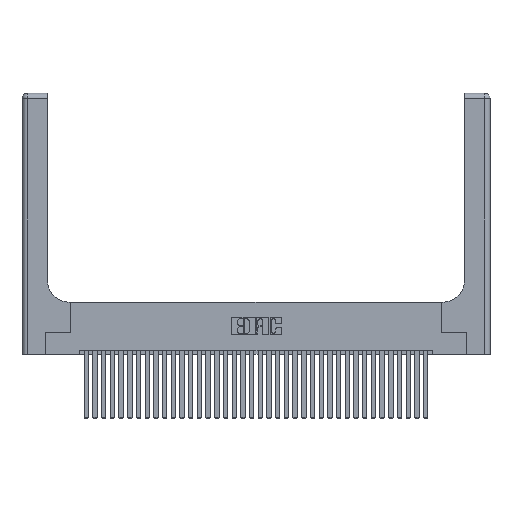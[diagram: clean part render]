
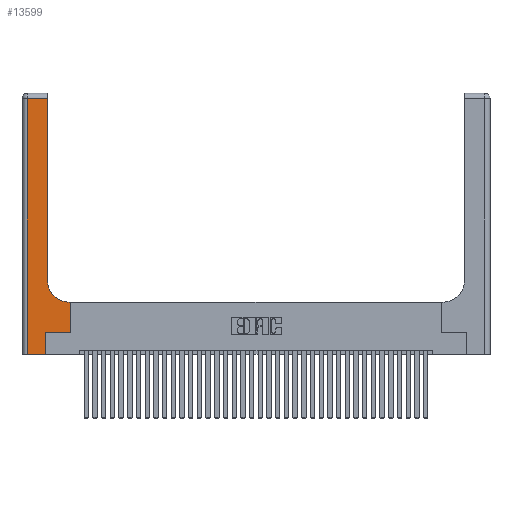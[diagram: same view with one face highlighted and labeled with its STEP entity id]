
A CAD part, top view. The second image highlights one B-rep face of the part: STEP entity #13599.
In plain terms, the highlighted planar face has unit normal (0, 0, 1).
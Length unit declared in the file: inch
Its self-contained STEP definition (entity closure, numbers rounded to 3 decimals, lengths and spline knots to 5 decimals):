
#496 = ORIENTED_EDGE ( 'NONE', *, *, #11008, .T. ) ;
#548 = CARTESIAN_POINT ( 'NONE',  ( 0.269, 0., 0.37 ) ) ;
#889 = CARTESIAN_POINT ( 'NONE',  ( 0.2915, 0.6, 0.37 ) ) ;
#1592 = LINE ( 'NONE', #29395, #14939 ) ;
#2134 = CARTESIAN_POINT ( 'NONE',  ( 0., 2.94, 0.37 ) ) ;
#2158 = EDGE_CURVE ( 'NONE', #29764, #23592, #24535, .T. ) ;
#2221 = PLANE ( 'NONE',  #5436 ) ;
#2252 = EDGE_CURVE ( 'NONE', #26574, #28063, #7174, .T. ) ;
#2369 = VECTOR ( 'NONE', #18025, 39.37008 ) ;
#3468 = CIRCLE ( 'NONE', #23201, 0.25 ) ;
#4026 = CARTESIAN_POINT ( 'NONE',  ( 0.06, 3., 0.37 ) ) ;
#4103 = DIRECTION ( 'NONE',  ( 1., 0., 0. ) ) ;
#4228 = CARTESIAN_POINT ( 'NONE',  ( 0.06, 2.94, 0.37 ) ) ;
#5436 = AXIS2_PLACEMENT_3D ( 'NONE', #36369, #20062, #33986 ) ;
#5738 = ORIENTED_EDGE ( 'NONE', *, *, #30671, .T. ) ;
#6675 = VECTOR ( 'NONE', #4103, 39.37008 ) ;
#7097 = LINE ( 'NONE', #4026, #28779 ) ;
#7174 = LINE ( 'NONE', #20875, #2369 ) ;
#7658 = EDGE_CURVE ( 'NONE', #34071, #34764, #11620, .T. ) ;
#7854 = LINE ( 'NONE', #889, #15300 ) ;
#8533 = LINE ( 'NONE', #22028, #33253 ) ;
#8614 = VECTOR ( 'NONE', #22234, 39.37008 ) ;
#9090 = CARTESIAN_POINT ( 'NONE',  ( 0.2915, 0.85, 0.37 ) ) ;
#9598 = LINE ( 'NONE', #2134, #13642 ) ;
#10315 = CARTESIAN_POINT ( 'NONE',  ( 0.2915, 2.94, 0.37 ) ) ;
#11008 = EDGE_CURVE ( 'NONE', #34764, #17682, #8533, .T. ) ;
#11620 = LINE ( 'NONE', #35247, #6675 ) ;
#11854 = EDGE_LOOP ( 'NONE', ( #35634, #26322, #27978, #12599, #496, #5738, #20880, #15048, #35899 ) ) ;
#12599 = ORIENTED_EDGE ( 'NONE', *, *, #7658, .T. ) ;
#13449 = EDGE_CURVE ( 'NONE', #21220, #26574, #3468, .T. ) ;
#13599 = ADVANCED_FACE ( 'NONE', ( #21659 ), #2221, .F. ) ;
#13642 = VECTOR ( 'NONE', #21987, 39.37008 ) ;
#14250 = DIRECTION ( 'NONE',  ( 1., 0., 0. ) ) ;
#14939 = VECTOR ( 'NONE', #23418, 39.37008 ) ;
#15048 = ORIENTED_EDGE ( 'NONE', *, *, #19460, .T. ) ;
#15300 = VECTOR ( 'NONE', #23321, 39.37008 ) ;
#16754 = CARTESIAN_POINT ( 'NONE',  ( 0.06, 0., 0.37 ) ) ;
#16820 = VERTEX_POINT ( 'NONE', #4228 ) ;
#17682 = VERTEX_POINT ( 'NONE', #31981 ) ;
#18025 = DIRECTION ( 'NONE',  ( 0., 1., 0. ) ) ;
#19460 = EDGE_CURVE ( 'NONE', #23592, #21220, #7854, .T. ) ;
#20062 = DIRECTION ( 'NONE',  ( 0., 0., -1. ) ) ;
#20875 = CARTESIAN_POINT ( 'NONE',  ( 0.2915, 3., 0.37 ) ) ;
#20880 = ORIENTED_EDGE ( 'NONE', *, *, #2158, .T. ) ;
#20883 = DIRECTION ( 'NONE',  ( 0., -1., 0. ) ) ;
#21220 = VERTEX_POINT ( 'NONE', #29720 ) ;
#21659 = FACE_OUTER_BOUND ( 'NONE', #11854, .T. ) ;
#21987 = DIRECTION ( 'NONE',  ( -1., 0., 0. ) ) ;
#22028 = CARTESIAN_POINT ( 'NONE',  ( 0.269, 0., 0.37 ) ) ;
#22234 = DIRECTION ( 'NONE',  ( 0., 1., 0. ) ) ;
#23201 = AXIS2_PLACEMENT_3D ( 'NONE', #31136, #34219, #14250 ) ;
#23321 = DIRECTION ( 'NONE',  ( -1., 0., 0. ) ) ;
#23418 = DIRECTION ( 'NONE',  ( 1., 0., 0. ) ) ;
#23592 = VERTEX_POINT ( 'NONE', #27093 ) ;
#24535 = LINE ( 'NONE', #33162, #8614 ) ;
#25059 = EDGE_CURVE ( 'NONE', #28063, #16820, #9598, .T. ) ;
#26322 = ORIENTED_EDGE ( 'NONE', *, *, #25059, .T. ) ;
#26574 = VERTEX_POINT ( 'NONE', #9090 ) ;
#26839 = DIRECTION ( 'NONE',  ( 0., 1., 0. ) ) ;
#27093 = CARTESIAN_POINT ( 'NONE',  ( 0.5585, 0.6, 0.37 ) ) ;
#27978 = ORIENTED_EDGE ( 'NONE', *, *, #28543, .T. ) ;
#28063 = VERTEX_POINT ( 'NONE', #10315 ) ;
#28543 = EDGE_CURVE ( 'NONE', #16820, #34071, #7097, .T. ) ;
#28779 = VECTOR ( 'NONE', #20883, 39.37008 ) ;
#29395 = CARTESIAN_POINT ( 'NONE',  ( 0.269, 0.25, 0.37 ) ) ;
#29720 = CARTESIAN_POINT ( 'NONE',  ( 0.5415, 0.6, 0.37 ) ) ;
#29764 = VERTEX_POINT ( 'NONE', #36581 ) ;
#30671 = EDGE_CURVE ( 'NONE', #17682, #29764, #1592, .T. ) ;
#31136 = CARTESIAN_POINT ( 'NONE',  ( 0.5415, 0.85, 0.37 ) ) ;
#31981 = CARTESIAN_POINT ( 'NONE',  ( 0.269, 0.25, 0.37 ) ) ;
#33162 = CARTESIAN_POINT ( 'NONE',  ( 0.5585, 0.25, 0.37 ) ) ;
#33253 = VECTOR ( 'NONE', #26839, 39.37008 ) ;
#33986 = DIRECTION ( 'NONE',  ( -1., 0., 0. ) ) ;
#34071 = VERTEX_POINT ( 'NONE', #16754 ) ;
#34219 = DIRECTION ( 'NONE',  ( 0., 0., -1. ) ) ;
#34764 = VERTEX_POINT ( 'NONE', #548 ) ;
#35247 = CARTESIAN_POINT ( 'NONE',  ( 0., 0., 0.37 ) ) ;
#35634 = ORIENTED_EDGE ( 'NONE', *, *, #2252, .T. ) ;
#35899 = ORIENTED_EDGE ( 'NONE', *, *, #13449, .T. ) ;
#36369 = CARTESIAN_POINT ( 'NONE',  ( 0., 3., 0.37 ) ) ;
#36581 = CARTESIAN_POINT ( 'NONE',  ( 0.5585, 0.25, 0.37 ) ) ;
